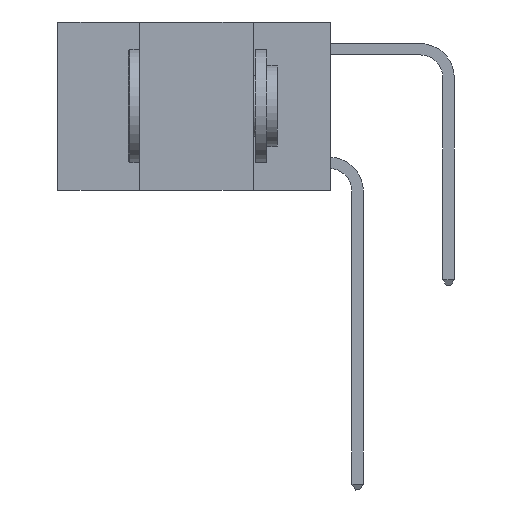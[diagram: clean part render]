
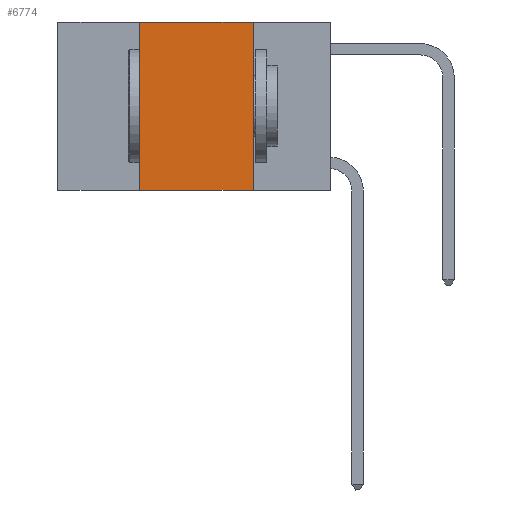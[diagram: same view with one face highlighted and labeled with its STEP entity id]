
A CAD part, left-side view. The second image highlights one B-rep face of the part: STEP entity #6774.
In plain terms, the highlighted planar face has unit normal (-1, 0, 0).
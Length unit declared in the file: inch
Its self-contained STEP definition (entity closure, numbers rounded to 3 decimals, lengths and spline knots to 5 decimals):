
#69 = CARTESIAN_POINT ( 'NONE',  ( 0., 0.6, -0.37 ) ) ;
#830 = EDGE_CURVE ( 'NONE', #2707, #6875, #13978, .T. ) ;
#1115 = DIRECTION ( 'NONE',  ( 0., 0., -1. ) ) ;
#1363 = CARTESIAN_POINT ( 'NONE',  ( 0., 0.42, 0. ) ) ;
#1381 = VECTOR ( 'NONE', #19332, 39.37008 ) ;
#1490 = CARTESIAN_POINT ( 'NONE',  ( 0., 0.17, 0. ) ) ;
#1806 = DIRECTION ( 'NONE',  ( 0., -1., 0. ) ) ;
#1956 = EDGE_CURVE ( 'NONE', #6341, #17577, #2763, .T. ) ;
#2437 = PLANE ( 'NONE',  #3650 ) ;
#2707 = VERTEX_POINT ( 'NONE', #3452 ) ;
#2763 = LINE ( 'NONE', #6012, #1381 ) ;
#2990 = DIRECTION ( 'NONE',  ( 0., 0., 1. ) ) ;
#3452 = CARTESIAN_POINT ( 'NONE',  ( 0., 0.42, -0.37 ) ) ;
#3650 = AXIS2_PLACEMENT_3D ( 'NONE', #5888, #13692, #1115 ) ;
#5552 = ORIENTED_EDGE ( 'NONE', *, *, #830, .T. ) ;
#5592 = CARTESIAN_POINT ( 'NONE',  ( 0., 0.17, -0.37 ) ) ;
#5888 = CARTESIAN_POINT ( 'NONE',  ( 0., 0.6, 0. ) ) ;
#6012 = CARTESIAN_POINT ( 'NONE',  ( 0., 0.6, 0. ) ) ;
#6341 = VERTEX_POINT ( 'NONE', #10691 ) ;
#6774 = ADVANCED_FACE ( 'NONE', ( #10567 ), #2437, .F. ) ;
#6875 = VERTEX_POINT ( 'NONE', #5592 ) ;
#6946 = ORIENTED_EDGE ( 'NONE', *, *, #1956, .F. ) ;
#9619 = EDGE_CURVE ( 'NONE', #17577, #6875, #18237, .T. ) ;
#10567 = FACE_OUTER_BOUND ( 'NONE', #11750, .T. ) ;
#10691 = CARTESIAN_POINT ( 'NONE',  ( 0., 0.42, 0. ) ) ;
#11750 = EDGE_LOOP ( 'NONE', ( #15304, #6946, #19183, #5552 ) ) ;
#12671 = VECTOR ( 'NONE', #1806, 39.37008 ) ;
#13633 = LINE ( 'NONE', #1363, #17762 ) ;
#13692 = DIRECTION ( 'NONE',  ( 1., 0., 0. ) ) ;
#13978 = LINE ( 'NONE', #69, #12671 ) ;
#15304 = ORIENTED_EDGE ( 'NONE', *, *, #9619, .F. ) ;
#15342 = VECTOR ( 'NONE', #16925, 39.37008 ) ;
#16925 = DIRECTION ( 'NONE',  ( 0., 0., -1. ) ) ;
#17557 = EDGE_CURVE ( 'NONE', #2707, #6341, #13633, .T. ) ;
#17577 = VERTEX_POINT ( 'NONE', #18610 ) ;
#17762 = VECTOR ( 'NONE', #2990, 39.37008 ) ;
#18237 = LINE ( 'NONE', #1490, #15342 ) ;
#18610 = CARTESIAN_POINT ( 'NONE',  ( 0., 0.17, 0. ) ) ;
#19183 = ORIENTED_EDGE ( 'NONE', *, *, #17557, .F. ) ;
#19332 = DIRECTION ( 'NONE',  ( 0., -1., 0. ) ) ;
